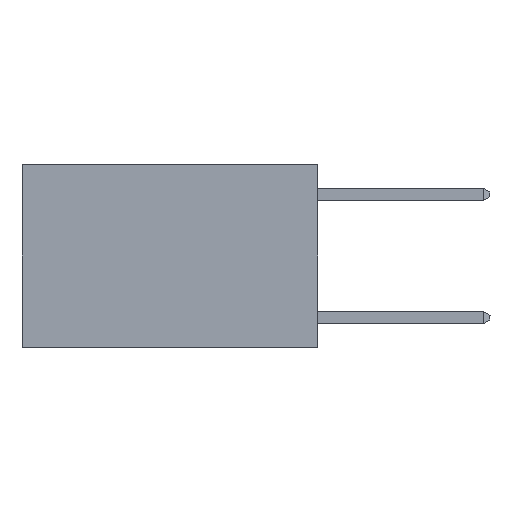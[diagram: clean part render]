
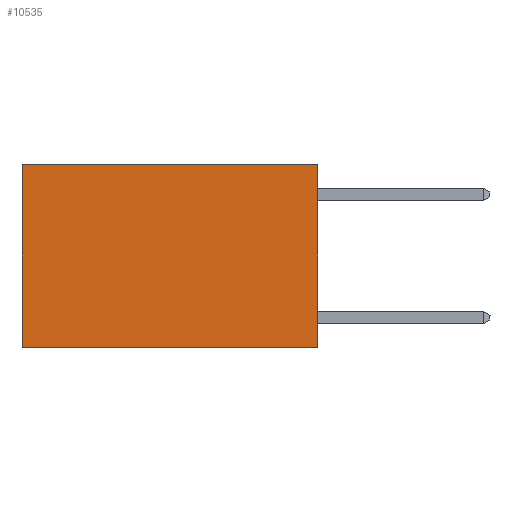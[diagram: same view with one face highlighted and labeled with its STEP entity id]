
A CAD part, left-side view. The second image highlights one B-rep face of the part: STEP entity #10535.
In plain terms, the highlighted planar face has unit normal (-1, 0, 0).
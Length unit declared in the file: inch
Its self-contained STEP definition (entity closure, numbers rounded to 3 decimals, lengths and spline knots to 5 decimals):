
#341 = CARTESIAN_POINT ( 'NONE',  ( 0.2625, 0., 0. ) ) ;
#1012 = LINE ( 'NONE', #14285, #22596 ) ;
#3346 = VECTOR ( 'NONE', #5214, 39.37008 ) ;
#4328 = EDGE_LOOP ( 'NONE', ( #7359, #15721, #20610, #7450 ) ) ;
#4575 = CARTESIAN_POINT ( 'NONE',  ( 0.2625, 0.6, -0.37 ) ) ;
#4669 = DIRECTION ( 'NONE',  ( 0., 1., 0. ) ) ;
#5214 = DIRECTION ( 'NONE',  ( 0., 0., -1. ) ) ;
#5458 = EDGE_CURVE ( 'NONE', #8379, #16456, #13811, .T. ) ;
#5935 = EDGE_CURVE ( 'NONE', #18845, #16456, #9803, .T. ) ;
#6111 = DIRECTION ( 'NONE',  ( 0., 1., 0. ) ) ;
#7359 = ORIENTED_EDGE ( 'NONE', *, *, #5935, .T. ) ;
#7450 = ORIENTED_EDGE ( 'NONE', *, *, #16523, .T. ) ;
#7868 = DIRECTION ( 'NONE',  ( 0., 0., -1. ) ) ;
#8379 = VERTEX_POINT ( 'NONE', #25704 ) ;
#9803 = LINE ( 'NONE', #20286, #3346 ) ;
#10147 = CARTESIAN_POINT ( 'NONE',  ( 0.2625, 0., 0. ) ) ;
#10471 = EDGE_CURVE ( 'NONE', #25839, #8379, #1012, .T. ) ;
#10535 = ADVANCED_FACE ( 'NONE', ( #10590 ), #22921, .F. ) ;
#10590 = FACE_OUTER_BOUND ( 'NONE', #4328, .T. ) ;
#12312 = DIRECTION ( 'NONE',  ( 1., 0., 0. ) ) ;
#13666 = LINE ( 'NONE', #341, #24260 ) ;
#13811 = LINE ( 'NONE', #16866, #25056 ) ;
#14285 = CARTESIAN_POINT ( 'NONE',  ( 0.2625, 0., 0. ) ) ;
#15721 = ORIENTED_EDGE ( 'NONE', *, *, #5458, .F. ) ;
#16456 = VERTEX_POINT ( 'NONE', #4575 ) ;
#16523 = EDGE_CURVE ( 'NONE', #25839, #18845, #13666, .T. ) ;
#16866 = CARTESIAN_POINT ( 'NONE',  ( 0.2625, 0., -0.37 ) ) ;
#18845 = VERTEX_POINT ( 'NONE', #27045 ) ;
#19253 = AXIS2_PLACEMENT_3D ( 'NONE', #10147, #12312, #27060 ) ;
#20286 = CARTESIAN_POINT ( 'NONE',  ( 0.2625, 0.6, 0. ) ) ;
#20610 = ORIENTED_EDGE ( 'NONE', *, *, #10471, .F. ) ;
#22085 = CARTESIAN_POINT ( 'NONE',  ( 0.2625, 0., 0. ) ) ;
#22596 = VECTOR ( 'NONE', #7868, 39.37008 ) ;
#22921 = PLANE ( 'NONE',  #19253 ) ;
#24260 = VECTOR ( 'NONE', #4669, 39.37008 ) ;
#25056 = VECTOR ( 'NONE', #6111, 39.37008 ) ;
#25704 = CARTESIAN_POINT ( 'NONE',  ( 0.2625, 0., -0.37 ) ) ;
#25839 = VERTEX_POINT ( 'NONE', #22085 ) ;
#27045 = CARTESIAN_POINT ( 'NONE',  ( 0.2625, 0.6, 0. ) ) ;
#27060 = DIRECTION ( 'NONE',  ( 0., 0., -1. ) ) ;
